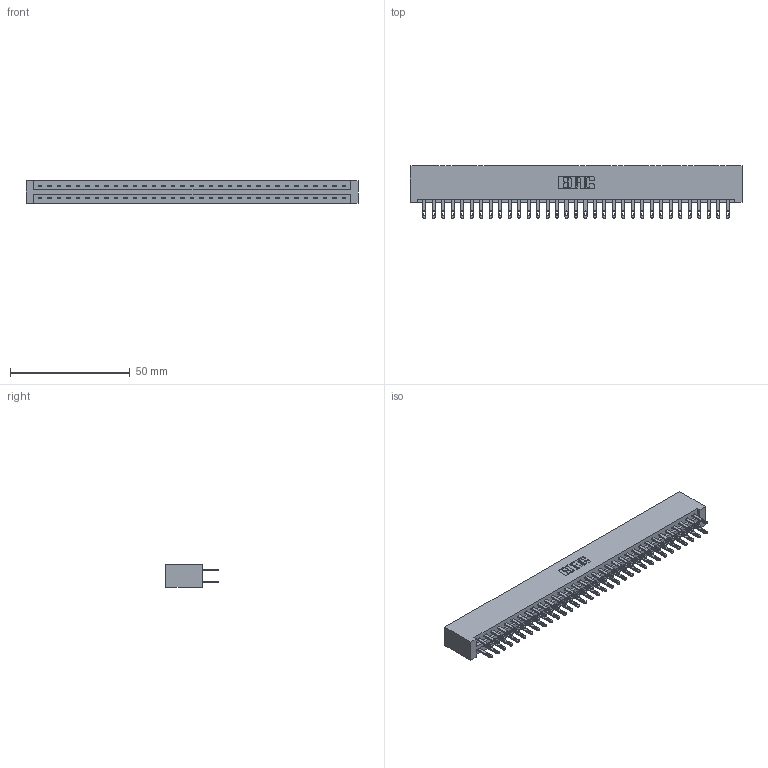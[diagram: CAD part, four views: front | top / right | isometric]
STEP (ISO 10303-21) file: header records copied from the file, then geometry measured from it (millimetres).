
FILE_DESCRIPTION (( 'STEP AP203' ), '1' );
FILE_NAME ('337-066-500-201.STEP', '2018-08-11T07:03:24', ( '' ), ( '' ), 'SwSTEP 2.0', 'SolidWorks 2016', '' );
FILE_SCHEMA (( 'CONFIG_CONTROL_DESIGN' ));
Length unit declared in the file: inch
Products named in the file (3): 337 Part_No Mounting Lugs; 345-292-001_345-293-100; 337-066-500-201
Assembly tree (67 placements, depth 2):
  337-066-500-201
    337 Part_No Mounting Lugs
    345-292-001_345-293-100  x66
Bounding box: 138.63 x 21.85 x 9.4 mm (x, y, z)
Volume: 15452.9 mm3; surface area: 18170.5 mm2
Topology: 67 solids, 67 shells, 3406 faces, 10385 edges, 6922 vertices
Faces by surface type: plane 2178, cylinder 1228
Entity records: 26403 total; most frequent: CARTESIAN_POINT 4454, ORIENTED_EDGE 4390, DIRECTION 3799, EDGE_CURVE 2195, VECTOR 2071, LINE 2071, VERTEX_POINT 1462, AXIS2_PLACEMENT_3D 864
